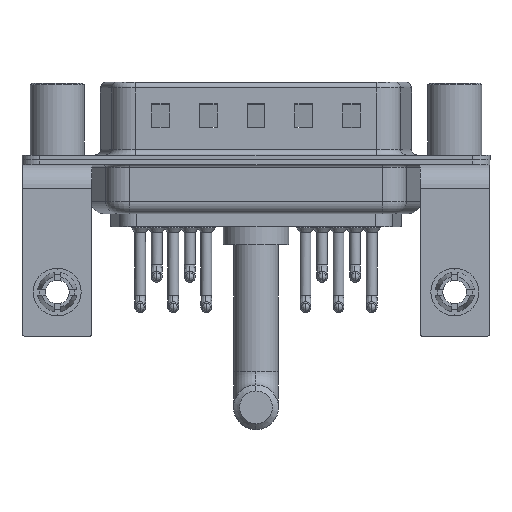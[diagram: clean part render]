
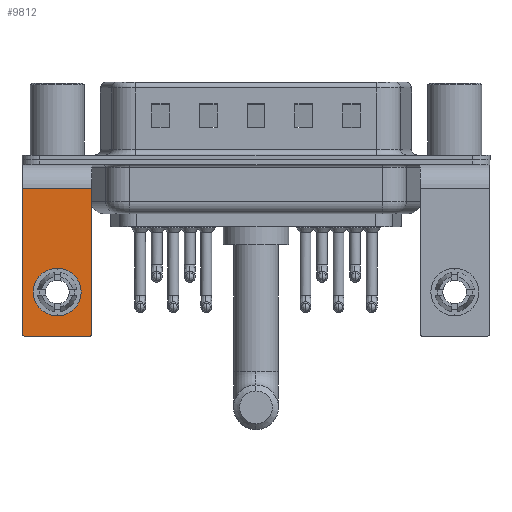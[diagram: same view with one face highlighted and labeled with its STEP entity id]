
A CAD part, front view. The second image highlights one B-rep face of the part: STEP entity #9812.
In plain terms, the highlighted planar face has unit normal (0, -1, 0).
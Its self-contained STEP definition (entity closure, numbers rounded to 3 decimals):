
#136 = CARTESIAN_POINT ( 'NONE',  ( -2.9, -6.25, -2.4 ) ) ;
#475 = CARTESIAN_POINT ( 'NONE',  ( 0., -6.25, -9.07 ) ) ;
#674 = CARTESIAN_POINT ( 'NONE',  ( 2.65, -6.25, -14.8 ) ) ;
#912 = VERTEX_POINT ( 'NONE', #24867 ) ;
#1169 = VERTEX_POINT ( 'NONE', #9830 ) ;
#1574 = DIRECTION ( 'NONE',  ( 0., 0., 1. ) ) ;
#1649 = PLANE ( 'NONE',  #7076 ) ;
#2372 = VECTOR ( 'NONE', #13625, 1000. ) ;
#3216 = VERTEX_POINT ( 'NONE', #674 ) ;
#3969 = DIRECTION ( 'NONE',  ( 0., -1., 0. ) ) ;
#4015 = CARTESIAN_POINT ( 'NONE',  ( -2.9, -6.25, -2.4 ) ) ;
#4676 = ORIENTED_EDGE ( 'NONE', *, *, #17921, .T. ) ;
#4754 = ORIENTED_EDGE ( 'NONE', *, *, #24647, .T. ) ;
#5729 = LINE ( 'NONE', #18332, #22818 ) ;
#6598 = VERTEX_POINT ( 'NONE', #10364 ) ;
#6920 = CARTESIAN_POINT ( 'NONE',  ( 0., -6.25, -13.07 ) ) ;
#7076 = AXIS2_PLACEMENT_3D ( 'NONE', #14351, #24293, #20405 ) ;
#7268 = DIRECTION ( 'NONE',  ( -1., 0., 0. ) ) ;
#7637 = VERTEX_POINT ( 'NONE', #475 ) ;
#7746 = DIRECTION ( 'NONE',  ( 0., 1., 0. ) ) ;
#7811 = ORIENTED_EDGE ( 'NONE', *, *, #10112, .T. ) ;
#7872 = VECTOR ( 'NONE', #7268, 1000. ) ;
#8183 = ORIENTED_EDGE ( 'NONE', *, *, #13723, .T. ) ;
#8320 = AXIS2_PLACEMENT_3D ( 'NONE', #11879, #7746, #1574 ) ;
#8384 = EDGE_LOOP ( 'NONE', ( #8183, #4676, #17423, #4754, #23176, #7811 ) ) ;
#9401 = EDGE_CURVE ( 'NONE', #15027, #7637, #19903, .T. ) ;
#9812 = ADVANCED_FACE ( 'NONE', ( #16103, #13951 ), #1649, .F. ) ;
#9830 = CARTESIAN_POINT ( 'NONE',  ( -2.65, -6.25, -14.8 ) ) ;
#10112 = EDGE_CURVE ( 'NONE', #6598, #19995, #19569, .T. ) ;
#10279 = CARTESIAN_POINT ( 'NONE',  ( -2.65, -6.25, -14.55 ) ) ;
#10364 = CARTESIAN_POINT ( 'NONE',  ( 2.9, -6.25, -2.4 ) ) ;
#11581 = ORIENTED_EDGE ( 'NONE', *, *, #16794, .T. ) ;
#11879 = CARTESIAN_POINT ( 'NONE',  ( 0., -6.25, -11.07 ) ) ;
#12819 = AXIS2_PLACEMENT_3D ( 'NONE', #10279, #3969, #24490 ) ;
#13416 = DIRECTION ( 'NONE',  ( 0., 1., 0. ) ) ;
#13625 = DIRECTION ( 'NONE',  ( -1., 0., 0. ) ) ;
#13723 = EDGE_CURVE ( 'NONE', #19995, #19073, #23870, .T. ) ;
#13845 = CIRCLE ( 'NONE', #14713, 0.25 ) ;
#13951 = FACE_OUTER_BOUND ( 'NONE', #8384, .T. ) ;
#14351 = CARTESIAN_POINT ( 'NONE',  ( 2.9, -6.25, -2.4 ) ) ;
#14713 = AXIS2_PLACEMENT_3D ( 'NONE', #20155, #22286, #22027 ) ;
#15027 = VERTEX_POINT ( 'NONE', #6920 ) ;
#15701 = VECTOR ( 'NONE', #16079, 1000. ) ;
#16079 = DIRECTION ( 'NONE',  ( 0., 0., -1. ) ) ;
#16103 = FACE_BOUND ( 'NONE', #20712, .T. ) ;
#16183 = AXIS2_PLACEMENT_3D ( 'NONE', #25657, #13416, #21758 ) ;
#16298 = DIRECTION ( 'NONE',  ( 0., 0., -1. ) ) ;
#16674 = CIRCLE ( 'NONE', #12819, 0.25 ) ;
#16794 = EDGE_CURVE ( 'NONE', #7637, #15027, #20084, .T. ) ;
#17423 = ORIENTED_EDGE ( 'NONE', *, *, #24925, .F. ) ;
#17921 = EDGE_CURVE ( 'NONE', #19073, #1169, #16674, .T. ) ;
#18332 = CARTESIAN_POINT ( 'NONE',  ( 2.9, -6.25, -2.4 ) ) ;
#18588 = ORIENTED_EDGE ( 'NONE', *, *, #9401, .T. ) ;
#19073 = VERTEX_POINT ( 'NONE', #24344 ) ;
#19215 = CARTESIAN_POINT ( 'NONE',  ( 2.9, -6.25, -14.8 ) ) ;
#19569 = LINE ( 'NONE', #25588, #2372 ) ;
#19903 = CIRCLE ( 'NONE', #8320, 2. ) ;
#19995 = VERTEX_POINT ( 'NONE', #136 ) ;
#20084 = CIRCLE ( 'NONE', #16183, 2. ) ;
#20155 = CARTESIAN_POINT ( 'NONE',  ( 2.65, -6.25, -14.55 ) ) ;
#20405 = DIRECTION ( 'NONE',  ( 0., 0., 1. ) ) ;
#20712 = EDGE_LOOP ( 'NONE', ( #18588, #11581 ) ) ;
#21070 = LINE ( 'NONE', #19215, #7872 ) ;
#21758 = DIRECTION ( 'NONE',  ( 0., 0., 1. ) ) ;
#22027 = DIRECTION ( 'NONE',  ( 0., 0., 1. ) ) ;
#22286 = DIRECTION ( 'NONE',  ( 0., -1., 0. ) ) ;
#22388 = EDGE_CURVE ( 'NONE', #6598, #912, #5729, .T. ) ;
#22818 = VECTOR ( 'NONE', #16298, 1000. ) ;
#23176 = ORIENTED_EDGE ( 'NONE', *, *, #22388, .F. ) ;
#23870 = LINE ( 'NONE', #4015, #15701 ) ;
#24293 = DIRECTION ( 'NONE',  ( 0., 1., 0. ) ) ;
#24344 = CARTESIAN_POINT ( 'NONE',  ( -2.9, -6.25, -14.55 ) ) ;
#24490 = DIRECTION ( 'NONE',  ( 0., 0., 1. ) ) ;
#24647 = EDGE_CURVE ( 'NONE', #3216, #912, #13845, .T. ) ;
#24867 = CARTESIAN_POINT ( 'NONE',  ( 2.9, -6.25, -14.55 ) ) ;
#24925 = EDGE_CURVE ( 'NONE', #3216, #1169, #21070, .T. ) ;
#25588 = CARTESIAN_POINT ( 'NONE',  ( 2.9, -6.25, -2.4 ) ) ;
#25657 = CARTESIAN_POINT ( 'NONE',  ( 0., -6.25, -11.07 ) ) ;
